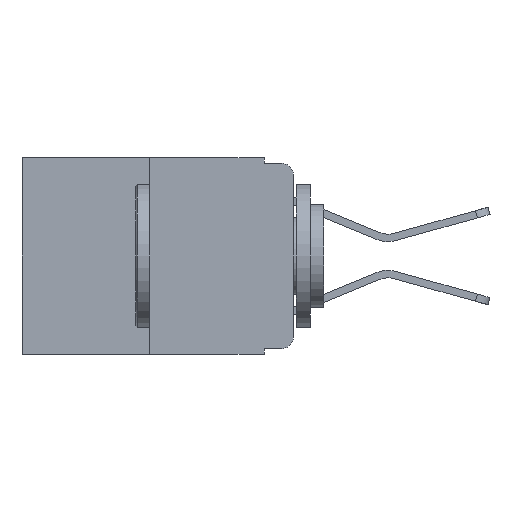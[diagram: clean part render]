
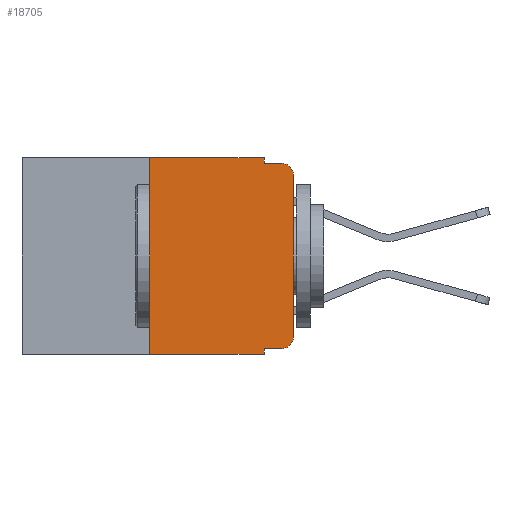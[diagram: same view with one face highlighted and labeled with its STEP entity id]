
A CAD part, left-side view. The second image highlights one B-rep face of the part: STEP entity #18705.
In plain terms, the highlighted planar face has unit normal (-1, 0, 0).
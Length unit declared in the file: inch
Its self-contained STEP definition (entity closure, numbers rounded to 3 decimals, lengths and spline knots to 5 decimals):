
#127 = CARTESIAN_POINT ( 'NONE',  ( 0., 0., -0.313 ) ) ;
#977 = VECTOR ( 'NONE', #19170, 39.37008 ) ;
#1396 = CARTESIAN_POINT ( 'NONE',  ( 0., 0.051, -0.01 ) ) ;
#2151 = ORIENTED_EDGE ( 'NONE', *, *, #14018, .T. ) ;
#2155 = VERTEX_POINT ( 'NONE', #4969 ) ;
#2497 = ORIENTED_EDGE ( 'NONE', *, *, #4311, .T. ) ;
#2706 = CARTESIAN_POINT ( 'NONE',  ( 0., 0.25, -0.343 ) ) ;
#2830 = EDGE_CURVE ( 'NONE', #16392, #21852, #19613, .T. ) ;
#3220 = DIRECTION ( 'NONE',  ( 1., 0., 0. ) ) ;
#3559 = LINE ( 'NONE', #3879, #18676 ) ;
#3879 = CARTESIAN_POINT ( 'NONE',  ( 0., 0.473, -0.343 ) ) ;
#4201 = ORIENTED_EDGE ( 'NONE', *, *, #9988, .F. ) ;
#4311 = EDGE_CURVE ( 'NONE', #9681, #16392, #17548, .T. ) ;
#4346 = CARTESIAN_POINT ( 'NONE',  ( 0., 0.25, 0. ) ) ;
#4885 = CARTESIAN_POINT ( 'NONE',  ( 0., 0.051, 0. ) ) ;
#4969 = CARTESIAN_POINT ( 'NONE',  ( 0., 0.051, -0.01 ) ) ;
#4998 = CARTESIAN_POINT ( 'NONE',  ( 0., 0.02, -0.333 ) ) ;
#5592 = DIRECTION ( 'NONE',  ( -1., 0., 0. ) ) ;
#5800 = EDGE_CURVE ( 'NONE', #9681, #6691, #7318, .T. ) ;
#6113 = LINE ( 'NONE', #4885, #977 ) ;
#6292 = ORIENTED_EDGE ( 'NONE', *, *, #18904, .T. ) ;
#6691 = VERTEX_POINT ( 'NONE', #15830 ) ;
#6746 = DIRECTION ( 'NONE',  ( 0., 0., -1. ) ) ;
#7318 = LINE ( 'NONE', #22898, #12080 ) ;
#7478 = PLANE ( 'NONE',  #24279 ) ;
#8045 = AXIS2_PLACEMENT_3D ( 'NONE', #17793, #5592, #19807 ) ;
#8366 = CARTESIAN_POINT ( 'NONE',  ( 0., 0., -0.03 ) ) ;
#8603 = EDGE_CURVE ( 'NONE', #11026, #15733, #23584, .T. ) ;
#9681 = VERTEX_POINT ( 'NONE', #20382 ) ;
#9849 = ORIENTED_EDGE ( 'NONE', *, *, #17907, .F. ) ;
#9988 = EDGE_CURVE ( 'NONE', #22016, #2155, #6113, .T. ) ;
#10075 = CARTESIAN_POINT ( 'NONE',  ( 0., 0.473, 0. ) ) ;
#10455 = ORIENTED_EDGE ( 'NONE', *, *, #8603, .F. ) ;
#10567 = VECTOR ( 'NONE', #15954, 39.37008 ) ;
#11026 = VERTEX_POINT ( 'NONE', #2706 ) ;
#11289 = EDGE_CURVE ( 'NONE', #2155, #14625, #15933, .T. ) ;
#12019 = ORIENTED_EDGE ( 'NONE', *, *, #15357, .T. ) ;
#12080 = VECTOR ( 'NONE', #6746, 39.37008 ) ;
#12762 = CARTESIAN_POINT ( 'NONE',  ( 0., 0.051, -0.333 ) ) ;
#13010 = FACE_OUTER_BOUND ( 'NONE', #24272, .T. ) ;
#14018 = EDGE_CURVE ( 'NONE', #18971, #14625, #18611, .T. ) ;
#14128 = DIRECTION ( 'NONE',  ( 0., -1., 0. ) ) ;
#14625 = VERTEX_POINT ( 'NONE', #15554 ) ;
#14763 = DIRECTION ( 'NONE',  ( -1., 0., 0. ) ) ;
#14902 = DIRECTION ( 'NONE',  ( 0., 0., -1. ) ) ;
#15357 = EDGE_CURVE ( 'NONE', #21852, #18971, #17905, .T. ) ;
#15554 = CARTESIAN_POINT ( 'NONE',  ( 0., 0.02, -0.01 ) ) ;
#15733 = VERTEX_POINT ( 'NONE', #4346 ) ;
#15753 = VECTOR ( 'NONE', #14128, 39.37008 ) ;
#15830 = CARTESIAN_POINT ( 'NONE',  ( 0., 0.051, -0.343 ) ) ;
#15933 = LINE ( 'NONE', #1396, #10567 ) ;
#15954 = DIRECTION ( 'NONE',  ( 0., -1., 0. ) ) ;
#16386 = LINE ( 'NONE', #10075, #15753 ) ;
#16392 = VERTEX_POINT ( 'NONE', #4998 ) ;
#17433 = CARTESIAN_POINT ( 'NONE',  ( 0., 0.051, 0. ) ) ;
#17548 = LINE ( 'NONE', #12762, #18804 ) ;
#17653 = DIRECTION ( 'NONE',  ( 0., 0., -1. ) ) ;
#17654 = VECTOR ( 'NONE', #23110, 39.37008 ) ;
#17793 = CARTESIAN_POINT ( 'NONE',  ( 0., 0.02, -0.03 ) ) ;
#17905 = LINE ( 'NONE', #25947, #22624 ) ;
#17907 = EDGE_CURVE ( 'NONE', #15733, #22016, #16386, .T. ) ;
#17978 = DIRECTION ( 'NONE',  ( 0., 0., 1. ) ) ;
#18611 = CIRCLE ( 'NONE', #8045, 0.02 ) ;
#18669 = AXIS2_PLACEMENT_3D ( 'NONE', #19959, #14763, #14902 ) ;
#18676 = VECTOR ( 'NONE', #22295, 39.37008 ) ;
#18705 = ADVANCED_FACE ( 'NONE', ( #13010 ), #7478, .F. ) ;
#18804 = VECTOR ( 'NONE', #24760, 39.37008 ) ;
#18904 = EDGE_CURVE ( 'NONE', #11026, #6691, #3559, .T. ) ;
#18971 = VERTEX_POINT ( 'NONE', #8366 ) ;
#19170 = DIRECTION ( 'NONE',  ( 0., 0., -1. ) ) ;
#19262 = ORIENTED_EDGE ( 'NONE', *, *, #11289, .F. ) ;
#19578 = CARTESIAN_POINT ( 'NONE',  ( 0., 0.473, 0. ) ) ;
#19613 = CIRCLE ( 'NONE', #18669, 0.02 ) ;
#19807 = DIRECTION ( 'NONE',  ( 0., 0., -1. ) ) ;
#19959 = CARTESIAN_POINT ( 'NONE',  ( 0., 0.02, -0.313 ) ) ;
#20382 = CARTESIAN_POINT ( 'NONE',  ( 0., 0.051, -0.333 ) ) ;
#21852 = VERTEX_POINT ( 'NONE', #127 ) ;
#22016 = VERTEX_POINT ( 'NONE', #17433 ) ;
#22295 = DIRECTION ( 'NONE',  ( 0., -1., 0. ) ) ;
#22624 = VECTOR ( 'NONE', #17978, 39.37008 ) ;
#22898 = CARTESIAN_POINT ( 'NONE',  ( 0., 0.051, 0. ) ) ;
#23110 = DIRECTION ( 'NONE',  ( 0., 0., 1. ) ) ;
#23584 = LINE ( 'NONE', #25088, #17654 ) ;
#23655 = ORIENTED_EDGE ( 'NONE', *, *, #5800, .F. ) ;
#24272 = EDGE_LOOP ( 'NONE', ( #12019, #2151, #19262, #4201, #9849, #10455, #6292, #23655, #2497, #24532 ) ) ;
#24279 = AXIS2_PLACEMENT_3D ( 'NONE', #19578, #3220, #17653 ) ;
#24532 = ORIENTED_EDGE ( 'NONE', *, *, #2830, .T. ) ;
#24760 = DIRECTION ( 'NONE',  ( 0., -1., 0. ) ) ;
#25088 = CARTESIAN_POINT ( 'NONE',  ( 0., 0.25, 0. ) ) ;
#25947 = CARTESIAN_POINT ( 'NONE',  ( 0., 0., 0. ) ) ;
